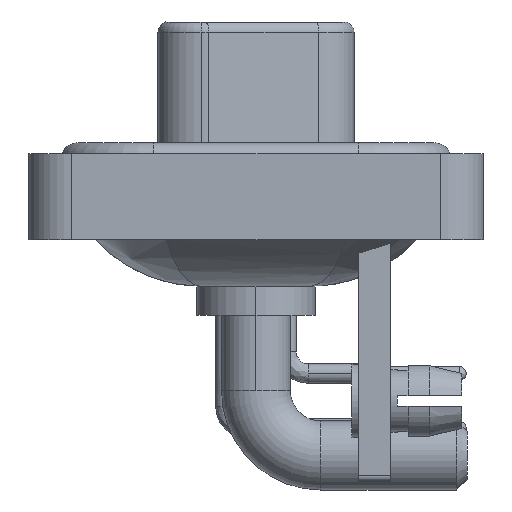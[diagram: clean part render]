
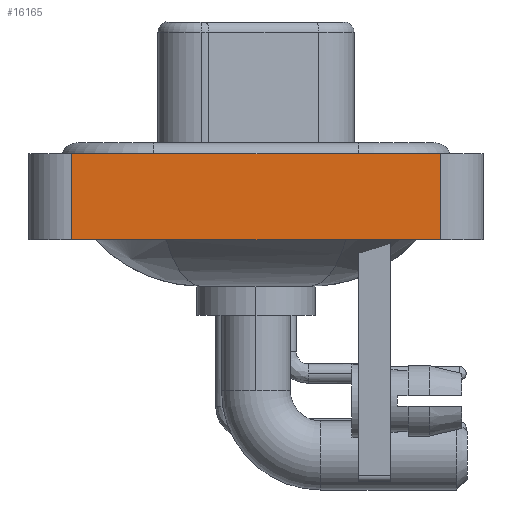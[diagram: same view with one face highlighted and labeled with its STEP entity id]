
A CAD part, left-side view. The second image highlights one B-rep face of the part: STEP entity #16165.
In plain terms, the highlighted planar face has unit normal (-1, 0, 0).
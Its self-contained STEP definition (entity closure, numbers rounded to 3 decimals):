
#511 = CARTESIAN_POINT ( 'NONE',  ( -7.3, 8.55, -3.6 ) ) ;
#548 = VECTOR ( 'NONE', #25507, 1000. ) ;
#976 = CARTESIAN_POINT ( 'NONE',  ( -7.3, -8.55, 0.4 ) ) ;
#2916 = EDGE_CURVE ( 'NONE', #13249, #4089, #18997, .T. ) ;
#3441 = DIRECTION ( 'NONE',  ( 0., -1., 0. ) ) ;
#4089 = VERTEX_POINT ( 'NONE', #19582 ) ;
#5924 = VERTEX_POINT ( 'NONE', #21945 ) ;
#6578 = DIRECTION ( 'NONE',  ( 0., 0., 1. ) ) ;
#6708 = VECTOR ( 'NONE', #3441, 1000. ) ;
#6711 = CARTESIAN_POINT ( 'NONE',  ( -7.3, -8.55, -3.6 ) ) ;
#7016 = AXIS2_PLACEMENT_3D ( 'NONE', #11540, #20155, #24130 ) ;
#7022 = VECTOR ( 'NONE', #6578, 1000. ) ;
#7332 = PLANE ( 'NONE',  #7016 ) ;
#8355 = EDGE_LOOP ( 'NONE', ( #18361, #25953, #18951, #26422 ) ) ;
#10556 = EDGE_CURVE ( 'NONE', #5924, #4089, #25769, .T. ) ;
#11540 = CARTESIAN_POINT ( 'NONE',  ( -7.3, -8.55, -3.6 ) ) ;
#11982 = EDGE_CURVE ( 'NONE', #15505, #13249, #16204, .T. ) ;
#12414 = VECTOR ( 'NONE', #19018, 1000. ) ;
#13249 = VERTEX_POINT ( 'NONE', #20021 ) ;
#15505 = VERTEX_POINT ( 'NONE', #17791 ) ;
#15632 = FACE_OUTER_BOUND ( 'NONE', #8355, .T. ) ;
#16165 = ADVANCED_FACE ( 'NONE', ( #15632 ), #7332, .T. ) ;
#16204 = LINE ( 'NONE', #18001, #6708 ) ;
#17791 = CARTESIAN_POINT ( 'NONE',  ( -7.3, 8.55, -3.6 ) ) ;
#17800 = EDGE_CURVE ( 'NONE', #15505, #5924, #19408, .T. ) ;
#18001 = CARTESIAN_POINT ( 'NONE',  ( -7.3, -8.55, -3.6 ) ) ;
#18361 = ORIENTED_EDGE ( 'NONE', *, *, #2916, .T. ) ;
#18951 = ORIENTED_EDGE ( 'NONE', *, *, #17800, .F. ) ;
#18997 = LINE ( 'NONE', #6711, #7022 ) ;
#19018 = DIRECTION ( 'NONE',  ( 0., 0., 1. ) ) ;
#19408 = LINE ( 'NONE', #511, #12414 ) ;
#19582 = CARTESIAN_POINT ( 'NONE',  ( -7.3, -8.55, 0.4 ) ) ;
#20021 = CARTESIAN_POINT ( 'NONE',  ( -7.3, -8.55, -3.6 ) ) ;
#20155 = DIRECTION ( 'NONE',  ( -1., 0., 0. ) ) ;
#21945 = CARTESIAN_POINT ( 'NONE',  ( -7.3, 8.55, 0.4 ) ) ;
#24130 = DIRECTION ( 'NONE',  ( 0., 0., 1. ) ) ;
#25507 = DIRECTION ( 'NONE',  ( 0., -1., 0. ) ) ;
#25769 = LINE ( 'NONE', #976, #548 ) ;
#25953 = ORIENTED_EDGE ( 'NONE', *, *, #10556, .F. ) ;
#26422 = ORIENTED_EDGE ( 'NONE', *, *, #11982, .T. ) ;
